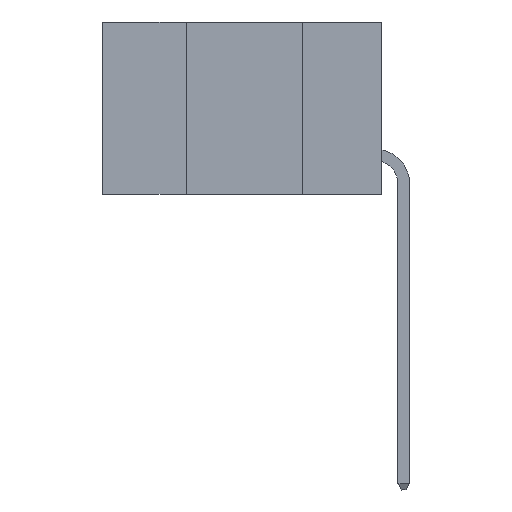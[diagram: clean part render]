
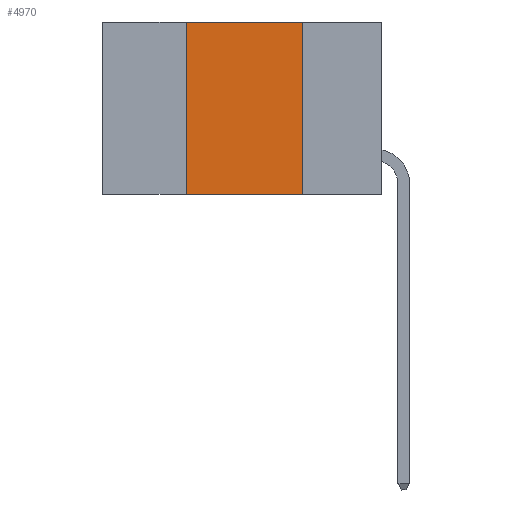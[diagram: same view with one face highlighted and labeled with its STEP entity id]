
A CAD part, left-side view. The second image highlights one B-rep face of the part: STEP entity #4970.
In plain terms, the highlighted planar face has unit normal (-1, 0, 0).
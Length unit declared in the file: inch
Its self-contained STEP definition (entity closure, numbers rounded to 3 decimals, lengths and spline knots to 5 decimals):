
#786 = DIRECTION ( 'NONE',  ( 0., -1., 0. ) ) ;
#950 = VECTOR ( 'NONE', #4837, 39.37008 ) ;
#2255 = CARTESIAN_POINT ( 'NONE',  ( 0., 0.42, 0. ) ) ;
#2401 = EDGE_CURVE ( 'NONE', #12852, #4135, #6281, .T. ) ;
#3270 = LINE ( 'NONE', #2255, #8584 ) ;
#3620 = CARTESIAN_POINT ( 'NONE',  ( 0., 0.17, 0. ) ) ;
#4135 = VERTEX_POINT ( 'NONE', #3620 ) ;
#4415 = LINE ( 'NONE', #4576, #950 ) ;
#4435 = EDGE_CURVE ( 'NONE', #4135, #10194, #4415, .T. ) ;
#4576 = CARTESIAN_POINT ( 'NONE',  ( 0., 0.17, 0. ) ) ;
#4599 = VERTEX_POINT ( 'NONE', #7219 ) ;
#4837 = DIRECTION ( 'NONE',  ( 0., 0., -1. ) ) ;
#4970 = ADVANCED_FACE ( 'NONE', ( #10090 ), #8905, .F. ) ;
#5116 = VECTOR ( 'NONE', #786, 39.37008 ) ;
#5170 = CARTESIAN_POINT ( 'NONE',  ( 0., 0.6, 0. ) ) ;
#5445 = LINE ( 'NONE', #7446, #5116 ) ;
#5832 = ORIENTED_EDGE ( 'NONE', *, *, #13487, .T. ) ;
#6281 = LINE ( 'NONE', #5170, #8717 ) ;
#6637 = AXIS2_PLACEMENT_3D ( 'NONE', #8026, #7618, #8457 ) ;
#6643 = DIRECTION ( 'NONE',  ( 0., 0., 1. ) ) ;
#6734 = DIRECTION ( 'NONE',  ( 0., -1., 0. ) ) ;
#7219 = CARTESIAN_POINT ( 'NONE',  ( 0., 0.42, -0.37 ) ) ;
#7270 = EDGE_CURVE ( 'NONE', #4599, #12852, #3270, .T. ) ;
#7446 = CARTESIAN_POINT ( 'NONE',  ( 0., 0.6, -0.37 ) ) ;
#7618 = DIRECTION ( 'NONE',  ( 1., 0., 0. ) ) ;
#8026 = CARTESIAN_POINT ( 'NONE',  ( 0., 0.6, 0. ) ) ;
#8112 = ORIENTED_EDGE ( 'NONE', *, *, #7270, .F. ) ;
#8283 = CARTESIAN_POINT ( 'NONE',  ( 0., 0.42, 0. ) ) ;
#8457 = DIRECTION ( 'NONE',  ( 0., 0., -1. ) ) ;
#8584 = VECTOR ( 'NONE', #6643, 39.37008 ) ;
#8717 = VECTOR ( 'NONE', #6734, 39.37008 ) ;
#8749 = EDGE_LOOP ( 'NONE', ( #11718, #11930, #8112, #5832 ) ) ;
#8905 = PLANE ( 'NONE',  #6637 ) ;
#9155 = CARTESIAN_POINT ( 'NONE',  ( 0., 0.17, -0.37 ) ) ;
#10090 = FACE_OUTER_BOUND ( 'NONE', #8749, .T. ) ;
#10194 = VERTEX_POINT ( 'NONE', #9155 ) ;
#11718 = ORIENTED_EDGE ( 'NONE', *, *, #4435, .F. ) ;
#11930 = ORIENTED_EDGE ( 'NONE', *, *, #2401, .F. ) ;
#12852 = VERTEX_POINT ( 'NONE', #8283 ) ;
#13487 = EDGE_CURVE ( 'NONE', #4599, #10194, #5445, .T. ) ;
